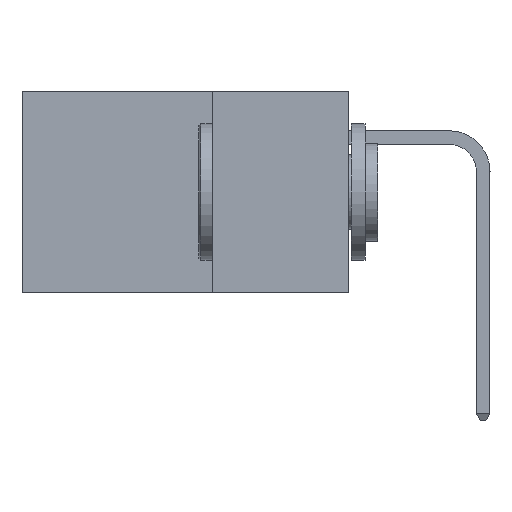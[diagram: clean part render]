
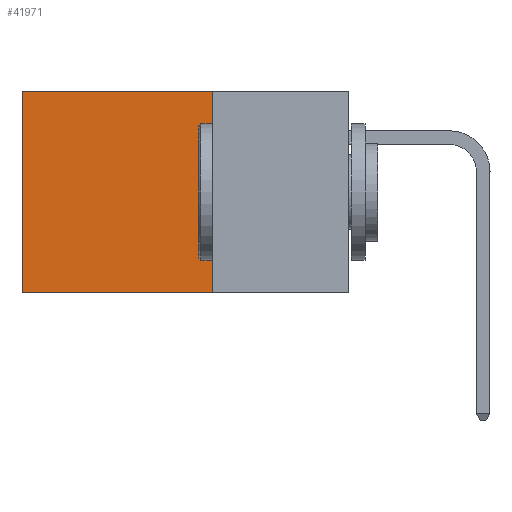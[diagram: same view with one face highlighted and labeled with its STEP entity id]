
A CAD part, left-side view. The second image highlights one B-rep face of the part: STEP entity #41971.
In plain terms, the highlighted planar face has unit normal (-1, 0, 0).
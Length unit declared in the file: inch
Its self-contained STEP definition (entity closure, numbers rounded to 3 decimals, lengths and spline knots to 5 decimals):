
#102 = VERTEX_POINT ( 'NONE', #11948 ) ;
#231 = LINE ( 'NONE', #32558, #38391 ) ;
#1386 = EDGE_CURVE ( 'NONE', #16483, #40529, #38376, .T. ) ;
#2403 = ORIENTED_EDGE ( 'NONE', *, *, #1386, .F. ) ;
#4121 = LINE ( 'NONE', #24657, #22650 ) ;
#6891 = DIRECTION ( 'NONE',  ( 0., 0., -1. ) ) ;
#7648 = VERTEX_POINT ( 'NONE', #30679 ) ;
#8067 = DIRECTION ( 'NONE',  ( 0., 0., -1. ) ) ;
#11530 = ORIENTED_EDGE ( 'NONE', *, *, #41284, .F. ) ;
#11948 = CARTESIAN_POINT ( 'NONE',  ( 0.2875, 0.6, 0. ) ) ;
#13853 = CARTESIAN_POINT ( 'NONE',  ( 0.2875, 0.6, -0.37 ) ) ;
#14812 = EDGE_CURVE ( 'NONE', #102, #40529, #231, .T. ) ;
#15074 = LINE ( 'NONE', #41466, #43291 ) ;
#16483 = VERTEX_POINT ( 'NONE', #17248 ) ;
#17248 = CARTESIAN_POINT ( 'NONE',  ( 0.2875, 0.25, -0.37 ) ) ;
#20287 = EDGE_LOOP ( 'NONE', ( #44620, #2403, #11530, #42811 ) ) ;
#20460 = CARTESIAN_POINT ( 'NONE',  ( 0.2875, 0.25, 0. ) ) ;
#22650 = VECTOR ( 'NONE', #32061, 39.37008 ) ;
#24171 = PLANE ( 'NONE',  #40229 ) ;
#24657 = CARTESIAN_POINT ( 'NONE',  ( 0.2875, 0.25, 0. ) ) ;
#26516 = CARTESIAN_POINT ( 'NONE',  ( 0.2875, 0.25, -0.37 ) ) ;
#27464 = VECTOR ( 'NONE', #30186, 39.37008 ) ;
#27902 = DIRECTION ( 'NONE',  ( 0., 0., -1. ) ) ;
#30186 = DIRECTION ( 'NONE',  ( 0., 1., 0. ) ) ;
#30679 = CARTESIAN_POINT ( 'NONE',  ( 0.2875, 0.25, 0. ) ) ;
#31738 = FACE_OUTER_BOUND ( 'NONE', #20287, .T. ) ;
#32061 = DIRECTION ( 'NONE',  ( 0., 1., 0. ) ) ;
#32558 = CARTESIAN_POINT ( 'NONE',  ( 0.2875, 0.6, 0. ) ) ;
#35108 = DIRECTION ( 'NONE',  ( 1., 0., 0. ) ) ;
#38376 = LINE ( 'NONE', #26516, #27464 ) ;
#38391 = VECTOR ( 'NONE', #6891, 39.37008 ) ;
#40229 = AXIS2_PLACEMENT_3D ( 'NONE', #20460, #35108, #27902 ) ;
#40485 = EDGE_CURVE ( 'NONE', #7648, #102, #4121, .T. ) ;
#40529 = VERTEX_POINT ( 'NONE', #13853 ) ;
#41284 = EDGE_CURVE ( 'NONE', #7648, #16483, #15074, .T. ) ;
#41466 = CARTESIAN_POINT ( 'NONE',  ( 0.2875, 0.25, 0. ) ) ;
#41971 = ADVANCED_FACE ( 'NONE', ( #31738 ), #24171, .F. ) ;
#42811 = ORIENTED_EDGE ( 'NONE', *, *, #40485, .T. ) ;
#43291 = VECTOR ( 'NONE', #8067, 39.37008 ) ;
#44620 = ORIENTED_EDGE ( 'NONE', *, *, #14812, .T. ) ;
